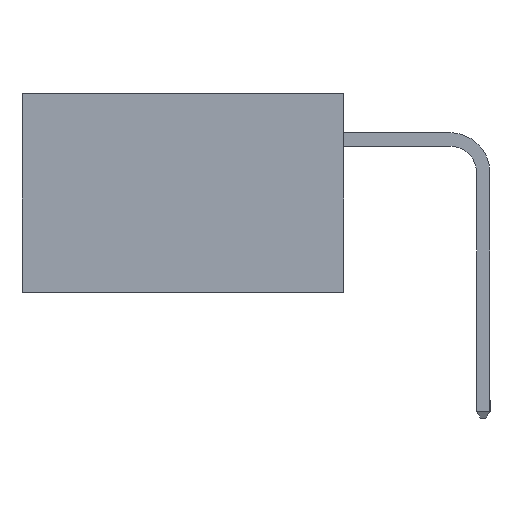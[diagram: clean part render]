
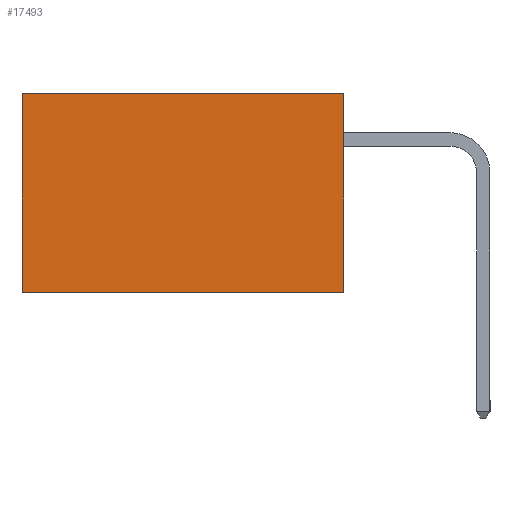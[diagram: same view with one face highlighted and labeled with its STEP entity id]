
A CAD part, left-side view. The second image highlights one B-rep face of the part: STEP entity #17493.
In plain terms, the highlighted planar face has unit normal (-1, 0, 0).
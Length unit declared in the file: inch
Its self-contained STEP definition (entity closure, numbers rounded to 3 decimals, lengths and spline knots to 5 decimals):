
#548 = CARTESIAN_POINT ( 'NONE',  ( 0.2615, 0.6, -0.37 ) ) ;
#1341 = FACE_OUTER_BOUND ( 'NONE', #2450, .T. ) ;
#1521 = ORIENTED_EDGE ( 'NONE', *, *, #14316, .T. ) ;
#1548 = DIRECTION ( 'NONE',  ( 0., 1., 0. ) ) ;
#2450 = EDGE_LOOP ( 'NONE', ( #21757, #12504, #19295, #1521 ) ) ;
#3111 = VERTEX_POINT ( 'NONE', #3653 ) ;
#3653 = CARTESIAN_POINT ( 'NONE',  ( 0.2615, 0.6, 0. ) ) ;
#3791 = DIRECTION ( 'NONE',  ( 0., 0., -1. ) ) ;
#6879 = LINE ( 'NONE', #21886, #20783 ) ;
#7762 = VECTOR ( 'NONE', #11925, 39.37008 ) ;
#7985 = DIRECTION ( 'NONE',  ( 0., 0., -1. ) ) ;
#8906 = VECTOR ( 'NONE', #1548, 39.37008 ) ;
#9398 = EDGE_CURVE ( 'NONE', #11327, #22994, #11408, .T. ) ;
#9614 = DIRECTION ( 'NONE',  ( 0., 1., 0. ) ) ;
#10896 = CARTESIAN_POINT ( 'NONE',  ( 0.2615, 0., -0.37 ) ) ;
#11327 = VERTEX_POINT ( 'NONE', #22719 ) ;
#11408 = LINE ( 'NONE', #10896, #13435 ) ;
#11925 = DIRECTION ( 'NONE',  ( 0., 0., -1. ) ) ;
#12504 = ORIENTED_EDGE ( 'NONE', *, *, #9398, .F. ) ;
#12528 = CARTESIAN_POINT ( 'NONE',  ( 0.2615, 0., 0. ) ) ;
#12630 = LINE ( 'NONE', #20937, #7762 ) ;
#13435 = VECTOR ( 'NONE', #9614, 39.37008 ) ;
#14316 = EDGE_CURVE ( 'NONE', #21264, #3111, #23318, .T. ) ;
#14867 = AXIS2_PLACEMENT_3D ( 'NONE', #17075, #18887, #7985 ) ;
#15094 = EDGE_CURVE ( 'NONE', #21264, #11327, #6879, .T. ) ;
#15259 = PLANE ( 'NONE',  #14867 ) ;
#17052 = CARTESIAN_POINT ( 'NONE',  ( 0.2615, 0., 0. ) ) ;
#17075 = CARTESIAN_POINT ( 'NONE',  ( 0.2615, 0., -0.37 ) ) ;
#17493 = ADVANCED_FACE ( 'NONE', ( #1341 ), #15259, .F. ) ;
#18887 = DIRECTION ( 'NONE',  ( 1., 0., 0. ) ) ;
#19295 = ORIENTED_EDGE ( 'NONE', *, *, #15094, .F. ) ;
#20783 = VECTOR ( 'NONE', #3791, 39.37008 ) ;
#20937 = CARTESIAN_POINT ( 'NONE',  ( 0.2615, 0.6, -0.37 ) ) ;
#21264 = VERTEX_POINT ( 'NONE', #17052 ) ;
#21757 = ORIENTED_EDGE ( 'NONE', *, *, #23104, .T. ) ;
#21886 = CARTESIAN_POINT ( 'NONE',  ( 0.2615, 0., -0.37 ) ) ;
#22719 = CARTESIAN_POINT ( 'NONE',  ( 0.2615, 0., -0.37 ) ) ;
#22994 = VERTEX_POINT ( 'NONE', #548 ) ;
#23104 = EDGE_CURVE ( 'NONE', #3111, #22994, #12630, .T. ) ;
#23318 = LINE ( 'NONE', #12528, #8906 ) ;
